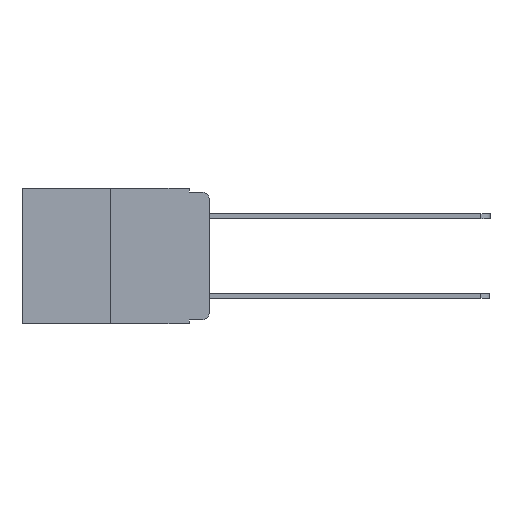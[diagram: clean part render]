
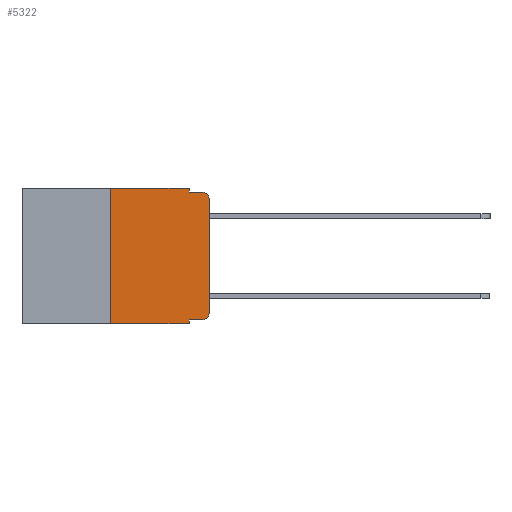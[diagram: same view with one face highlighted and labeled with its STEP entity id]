
A CAD part, left-side view. The second image highlights one B-rep face of the part: STEP entity #5322.
In plain terms, the highlighted planar face has unit normal (-1, 0, 0).
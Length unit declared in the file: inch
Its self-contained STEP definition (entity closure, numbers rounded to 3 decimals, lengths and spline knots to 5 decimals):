
#16 = ORIENTED_EDGE ( 'NONE', *, *, #21942, .T. ) ;
#78 = ORIENTED_EDGE ( 'NONE', *, *, #13411, .F. ) ;
#254 = VERTEX_POINT ( 'NONE', #18664 ) ;
#333 = ORIENTED_EDGE ( 'NONE', *, *, #16675, .F. ) ;
#542 = ORIENTED_EDGE ( 'NONE', *, *, #17924, .T. ) ;
#575 = ORIENTED_EDGE ( 'NONE', *, *, #10041, .T. ) ;
#843 = ORIENTED_EDGE ( 'NONE', *, *, #19053, .T. ) ;
#887 = CARTESIAN_POINT ( 'NONE',  ( 0., 0., -0.03 ) ) ;
#1030 = ORIENTED_EDGE ( 'NONE', *, *, #15682, .F. ) ;
#1450 = VERTEX_POINT ( 'NONE', #21687 ) ;
#1650 = DIRECTION ( 'NONE',  ( 0., 0., -1. ) ) ;
#1822 = VECTOR ( 'NONE', #15957, 39.37008 ) ;
#1940 = AXIS2_PLACEMENT_3D ( 'NONE', #20383, #10365, #9548 ) ;
#2325 = DIRECTION ( 'NONE',  ( 0., 0., 1. ) ) ;
#2936 = EDGE_LOOP ( 'NONE', ( #843, #542, #1030, #3655, #333, #78, #16, #10843, #3086, #575 ) ) ;
#3086 = ORIENTED_EDGE ( 'NONE', *, *, #11158, .T. ) ;
#3277 = VERTEX_POINT ( 'NONE', #4474 ) ;
#3328 = CARTESIAN_POINT ( 'NONE',  ( 0., 0.051, 0. ) ) ;
#3494 = CARTESIAN_POINT ( 'NONE',  ( 0., 0.02, -0.313 ) ) ;
#3655 = ORIENTED_EDGE ( 'NONE', *, *, #14512, .F. ) ;
#4146 = VECTOR ( 'NONE', #9259, 39.37008 ) ;
#4474 = CARTESIAN_POINT ( 'NONE',  ( 0., 0.051, -0.01 ) ) ;
#4732 = LINE ( 'NONE', #15949, #4146 ) ;
#4911 = CIRCLE ( 'NONE', #8164, 0.02 ) ;
#5107 = CARTESIAN_POINT ( 'NONE',  ( 0., 0.25, -0.343 ) ) ;
#5265 = DIRECTION ( 'NONE',  ( 0., 0., -1. ) ) ;
#5322 = ADVANCED_FACE ( 'NONE', ( #13799 ), #15274, .F. ) ;
#6097 = VERTEX_POINT ( 'NONE', #18224 ) ;
#6298 = VECTOR ( 'NONE', #20061, 39.37008 ) ;
#6510 = VECTOR ( 'NONE', #19245, 39.37008 ) ;
#6718 = CARTESIAN_POINT ( 'NONE',  ( 0., 0.051, -0.333 ) ) ;
#6832 = LINE ( 'NONE', #18401, #6298 ) ;
#7683 = VECTOR ( 'NONE', #1650, 39.37008 ) ;
#7857 = LINE ( 'NONE', #20135, #16293 ) ;
#8164 = AXIS2_PLACEMENT_3D ( 'NONE', #3494, #15373, #5265 ) ;
#8578 = DIRECTION ( 'NONE',  ( 0., 0., -1. ) ) ;
#8615 = CARTESIAN_POINT ( 'NONE',  ( 0., 0.473, -0.343 ) ) ;
#9259 = DIRECTION ( 'NONE',  ( 0., -1., 0. ) ) ;
#9548 = DIRECTION ( 'NONE',  ( 0., 0., -1. ) ) ;
#9589 = VECTOR ( 'NONE', #10304, 39.37008 ) ;
#10041 = EDGE_CURVE ( 'NONE', #254, #1450, #4911, .T. ) ;
#10304 = DIRECTION ( 'NONE',  ( 0., -1., 0. ) ) ;
#10365 = DIRECTION ( 'NONE',  ( -1., 0., 0. ) ) ;
#10546 = CARTESIAN_POINT ( 'NONE',  ( 0., 0.473, 0. ) ) ;
#10720 = CARTESIAN_POINT ( 'NONE',  ( 0., 0.02, -0.01 ) ) ;
#10843 = ORIENTED_EDGE ( 'NONE', *, *, #12272, .F. ) ;
#10905 = VERTEX_POINT ( 'NONE', #14189 ) ;
#11076 = CIRCLE ( 'NONE', #1940, 0.02 ) ;
#11158 = EDGE_CURVE ( 'NONE', #17151, #254, #6832, .T. ) ;
#11402 = LINE ( 'NONE', #10546, #19794 ) ;
#11499 = LINE ( 'NONE', #14233, #6510 ) ;
#11873 = VERTEX_POINT ( 'NONE', #887 ) ;
#12272 = EDGE_CURVE ( 'NONE', #17151, #10905, #11499, .T. ) ;
#12684 = LINE ( 'NONE', #3328, #7683 ) ;
#13411 = EDGE_CURVE ( 'NONE', #20735, #20021, #15411, .T. ) ;
#13799 = FACE_OUTER_BOUND ( 'NONE', #2936, .T. ) ;
#14189 = CARTESIAN_POINT ( 'NONE',  ( 0., 0.051, -0.343 ) ) ;
#14233 = CARTESIAN_POINT ( 'NONE',  ( 0., 0.051, 0. ) ) ;
#14252 = CARTESIAN_POINT ( 'NONE',  ( 0., 0.25, 0. ) ) ;
#14512 = EDGE_CURVE ( 'NONE', #6097, #3277, #12684, .T. ) ;
#14999 = CARTESIAN_POINT ( 'NONE',  ( 0., 0.25, 0. ) ) ;
#15274 = PLANE ( 'NONE',  #16768 ) ;
#15373 = DIRECTION ( 'NONE',  ( -1., 0., 0. ) ) ;
#15411 = LINE ( 'NONE', #14252, #1822 ) ;
#15682 = EDGE_CURVE ( 'NONE', #3277, #20320, #4732, .T. ) ;
#15949 = CARTESIAN_POINT ( 'NONE',  ( 0., 0.051, -0.01 ) ) ;
#15957 = DIRECTION ( 'NONE',  ( 0., 0., 1. ) ) ;
#16293 = VECTOR ( 'NONE', #2325, 39.37008 ) ;
#16675 = EDGE_CURVE ( 'NONE', #20021, #6097, #11402, .T. ) ;
#16768 = AXIS2_PLACEMENT_3D ( 'NONE', #16966, #18658, #8578 ) ;
#16966 = CARTESIAN_POINT ( 'NONE',  ( 0., 0.473, 0. ) ) ;
#17151 = VERTEX_POINT ( 'NONE', #6718 ) ;
#17924 = EDGE_CURVE ( 'NONE', #11873, #20320, #11076, .T. ) ;
#18224 = CARTESIAN_POINT ( 'NONE',  ( 0., 0.051, 0. ) ) ;
#18401 = CARTESIAN_POINT ( 'NONE',  ( 0., 0.051, -0.333 ) ) ;
#18658 = DIRECTION ( 'NONE',  ( 1., 0., 0. ) ) ;
#18664 = CARTESIAN_POINT ( 'NONE',  ( 0., 0.02, -0.333 ) ) ;
#19053 = EDGE_CURVE ( 'NONE', #1450, #11873, #7857, .T. ) ;
#19064 = LINE ( 'NONE', #8615, #9589 ) ;
#19245 = DIRECTION ( 'NONE',  ( 0., 0., -1. ) ) ;
#19794 = VECTOR ( 'NONE', #20642, 39.37008 ) ;
#20021 = VERTEX_POINT ( 'NONE', #14999 ) ;
#20061 = DIRECTION ( 'NONE',  ( 0., -1., 0. ) ) ;
#20135 = CARTESIAN_POINT ( 'NONE',  ( 0., 0., 0. ) ) ;
#20320 = VERTEX_POINT ( 'NONE', #10720 ) ;
#20383 = CARTESIAN_POINT ( 'NONE',  ( 0., 0.02, -0.03 ) ) ;
#20642 = DIRECTION ( 'NONE',  ( 0., -1., 0. ) ) ;
#20735 = VERTEX_POINT ( 'NONE', #5107 ) ;
#21687 = CARTESIAN_POINT ( 'NONE',  ( 0., 0., -0.313 ) ) ;
#21942 = EDGE_CURVE ( 'NONE', #20735, #10905, #19064, .T. ) ;
